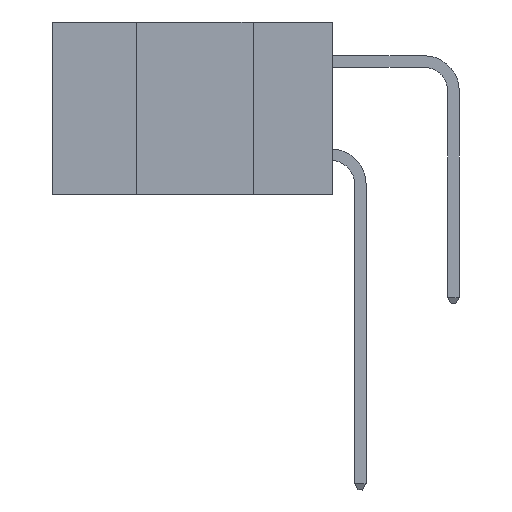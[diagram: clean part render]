
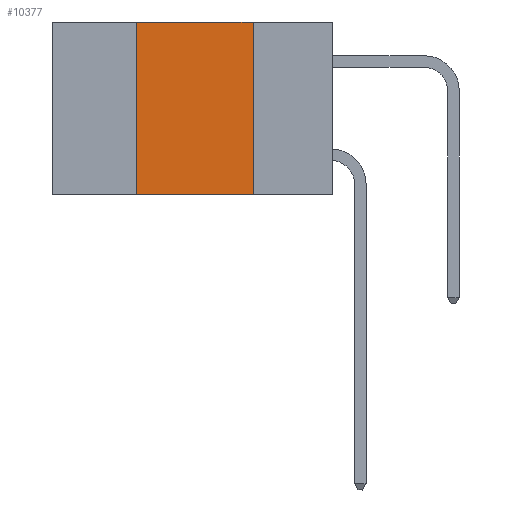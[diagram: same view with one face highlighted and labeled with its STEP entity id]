
A CAD part, left-side view. The second image highlights one B-rep face of the part: STEP entity #10377.
In plain terms, the highlighted planar face has unit normal (-1, 0, 0).
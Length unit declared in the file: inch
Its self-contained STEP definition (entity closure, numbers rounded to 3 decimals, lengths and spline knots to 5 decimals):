
#929 = CARTESIAN_POINT ( 'NONE',  ( 0., 0.6, -0.37 ) ) ;
#1188 = DIRECTION ( 'NONE',  ( 0., -1., 0. ) ) ;
#1585 = EDGE_CURVE ( 'NONE', #8272, #12408, #6431, .T. ) ;
#1914 = DIRECTION ( 'NONE',  ( 0., -1., 0. ) ) ;
#2364 = CARTESIAN_POINT ( 'NONE',  ( 0., 0.17, -0.37 ) ) ;
#2774 = EDGE_CURVE ( 'NONE', #13982, #15332, #8673, .T. ) ;
#2999 = DIRECTION ( 'NONE',  ( 0., 0., -1. ) ) ;
#3232 = EDGE_CURVE ( 'NONE', #15332, #8272, #14672, .T. ) ;
#3397 = PLANE ( 'NONE',  #7133 ) ;
#4500 = CARTESIAN_POINT ( 'NONE',  ( 0., 0.17, 0. ) ) ;
#4821 = VECTOR ( 'NONE', #2999, 39.37008 ) ;
#5337 = EDGE_LOOP ( 'NONE', ( #7549, #11559, #6447, #8295 ) ) ;
#5365 = CARTESIAN_POINT ( 'NONE',  ( 0., 0.17, -0.37 ) ) ;
#6009 = CARTESIAN_POINT ( 'NONE',  ( 0., 0.6, 0. ) ) ;
#6431 = LINE ( 'NONE', #5365, #4821 ) ;
#6447 = ORIENTED_EDGE ( 'NONE', *, *, #2774, .F. ) ;
#6934 = EDGE_CURVE ( 'NONE', #13982, #12408, #8296, .T. ) ;
#7133 = AXIS2_PLACEMENT_3D ( 'NONE', #15887, #13371, #13280 ) ;
#7549 = ORIENTED_EDGE ( 'NONE', *, *, #1585, .F. ) ;
#8272 = VERTEX_POINT ( 'NONE', #4500 ) ;
#8295 = ORIENTED_EDGE ( 'NONE', *, *, #6934, .T. ) ;
#8296 = LINE ( 'NONE', #929, #15692 ) ;
#8673 = LINE ( 'NONE', #10955, #10383 ) ;
#10377 = ADVANCED_FACE ( 'NONE', ( #12058 ), #3397, .F. ) ;
#10383 = VECTOR ( 'NONE', #13656, 39.37008 ) ;
#10931 = CARTESIAN_POINT ( 'NONE',  ( 0., 0.42, 0. ) ) ;
#10955 = CARTESIAN_POINT ( 'NONE',  ( 0., 0.42, -0.37 ) ) ;
#11452 = VECTOR ( 'NONE', #1188, 39.37008 ) ;
#11559 = ORIENTED_EDGE ( 'NONE', *, *, #3232, .F. ) ;
#12058 = FACE_OUTER_BOUND ( 'NONE', #5337, .T. ) ;
#12408 = VERTEX_POINT ( 'NONE', #2364 ) ;
#13280 = DIRECTION ( 'NONE',  ( 0., 0., -1. ) ) ;
#13371 = DIRECTION ( 'NONE',  ( 1., 0., 0. ) ) ;
#13656 = DIRECTION ( 'NONE',  ( 0., 0., 1. ) ) ;
#13982 = VERTEX_POINT ( 'NONE', #14607 ) ;
#14607 = CARTESIAN_POINT ( 'NONE',  ( 0., 0.42, -0.37 ) ) ;
#14672 = LINE ( 'NONE', #6009, #11452 ) ;
#15332 = VERTEX_POINT ( 'NONE', #10931 ) ;
#15692 = VECTOR ( 'NONE', #1914, 39.37008 ) ;
#15887 = CARTESIAN_POINT ( 'NONE',  ( 0., 0.6, 0. ) ) ;
